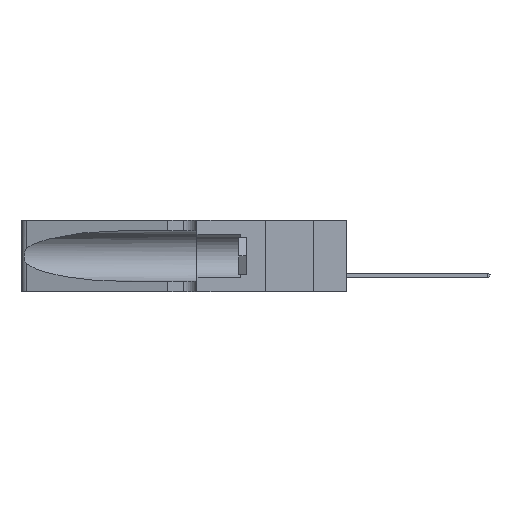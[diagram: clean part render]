
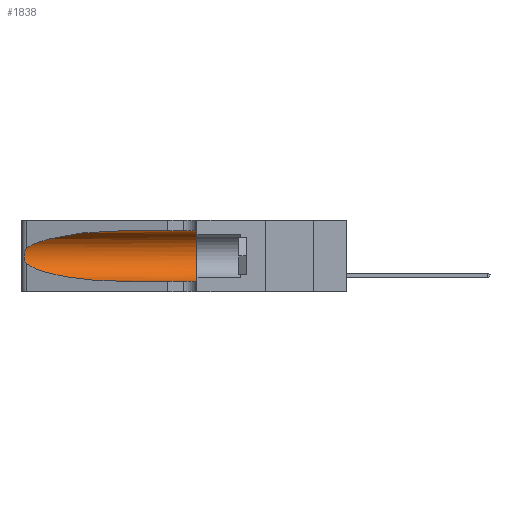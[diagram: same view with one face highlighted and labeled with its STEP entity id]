
A CAD part, left-side view. The second image highlights one B-rep face of the part: STEP entity #1838.
In plain terms, the highlighted cylindrical face has radius 3.308 mm (diameter 6.617 mm), a partial arc.
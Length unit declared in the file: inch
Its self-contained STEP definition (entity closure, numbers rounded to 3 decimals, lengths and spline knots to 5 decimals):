
#1838 = ADVANCED_FACE ( 'NONE', ( #8019 ), #14263, .F. ) ;
#2135 = ORIENTED_EDGE ( 'NONE', *, *, #30698, .F. ) ;
#2615 = CARTESIAN_POINT ( 'NONE',  ( 0.1305, 0.35, 0.05475 ) ) ;
#2997 = CARTESIAN_POINT ( 'NONE',  ( 0.25856, 1.23593, 0.16098 ) ) ;
#3150 = CARTESIAN_POINT ( 'NONE',  ( 0.25854, 1.2359, 0.20912 ) ) ;
#4646 = EDGE_CURVE ( 'NONE', #18827, #30359, #43256, .T. ) ;
#5749 = CARTESIAN_POINT ( 'NONE',  ( 0.25487, 1.22718, 0.22369 ) ) ;
#6407 = VERTEX_POINT ( 'NONE', #25254 ) ;
#6490 = CARTESIAN_POINT ( 'NONE',  ( 0.26075, 1.23896, 0.178 ) ) ;
#8019 = FACE_OUTER_BOUND ( 'NONE', #14316, .T. ) ;
#8082 = CARTESIAN_POINT ( 'NONE',  ( 0.25487, 1.22718, 0.22369 ) ) ;
#8113 = AXIS2_PLACEMENT_3D ( 'NONE', #31915, #13191, #38777 ) ;
#9425 = AXIS2_PLACEMENT_3D ( 'NONE', #25119, #47332, #36017 ) ;
#9522 = VERTEX_POINT ( 'NONE', #5749 ) ;
#11217 = VERTEX_POINT ( 'NONE', #24710 ) ;
#13018 = CARTESIAN_POINT ( 'NONE',  ( 0.25555, 1.22994, 0.2215 ) ) ;
#13031 = CARTESIAN_POINT ( 'NONE',  ( 0.25487, 1.22718, 0.14631 ) ) ;
#13191 = DIRECTION ( 'NONE',  ( 0., 1., 0. ) ) ;
#13321 = CARTESIAN_POINT ( 'NONE',  ( 0.25639, 1.23184, 0.21858 ) ) ;
#13982 = EDGE_CURVE ( 'NONE', #30359, #43902, #23854, .T. ) ;
#14232 =( BOUNDED_CURVE ( )  B_SPLINE_CURVE ( 3, ( #33499, #15241, #44472, #8082 ),
 .UNSPECIFIED., .F., .F. ) 
 B_SPLINE_CURVE_WITH_KNOTS ( ( 4, 4 ),
 ( 1.5708, 2.84003 ),
 .UNSPECIFIED. ) 
 CURVE ( )  GEOMETRIC_REPRESENTATION_ITEM ( )  RATIONAL_B_SPLINE_CURVE ( ( 1., 0.87, 0.87, 1. ) ) 
 REPRESENTATION_ITEM ( '' )  );
#14263 = CYLINDRICAL_SURFACE ( 'NONE', #9425, 0.13025 ) ;
#14316 = EDGE_LOOP ( 'NONE', ( #47153, #45351, #39743, #26605, #2135, #43108 ) ) ;
#15241 = CARTESIAN_POINT ( 'NONE',  ( 0.18966, 0.96281, 0.31525 ) ) ;
#16699 = CARTESIAN_POINT ( 'NONE',  ( 0.18966, 0.96281, 0.05475 ) ) ;
#17005 = CARTESIAN_POINT ( 'NONE',  ( 0.25789, 1.23486, 0.15765 ) ) ;
#17458 = CARTESIAN_POINT ( 'NONE',  ( 0.25487, 1.22718, 0.14631 ) ) ;
#17512 = DIRECTION ( 'NONE',  ( 0., -1., 0. ) ) ;
#18252 = EDGE_CURVE ( 'NONE', #11217, #9522, #14232, .T. ) ;
#18827 = VERTEX_POINT ( 'NONE', #34631 ) ;
#19654 = CIRCLE ( 'NONE', #8113, 0.13025 ) ;
#19898 = CARTESIAN_POINT ( 'NONE',  ( 0.25487, 1.22718, 0.22369 ) ) ;
#20819 = CARTESIAN_POINT ( 'NONE',  ( 0.25555, 1.22993, 0.14849 ) ) ;
#23854 = LINE ( 'NONE', #30295, #34180 ) ;
#24710 = CARTESIAN_POINT ( 'NONE',  ( 0.1305, 0.72297, 0.31525 ) ) ;
#25119 = CARTESIAN_POINT ( 'NONE',  ( 0.1305, 1.61858, 0.185 ) ) ;
#25254 = CARTESIAN_POINT ( 'NONE',  ( 0.1305, 0.35, 0.31525 ) ) ;
#26605 = ORIENTED_EDGE ( 'NONE', *, *, #13982, .T. ) ;
#28659 = CARTESIAN_POINT ( 'NONE',  ( 0.25639, 1.23186, 0.15144 ) ) ;
#28891 = CARTESIAN_POINT ( 'NONE',  ( 0.1305, 1.61858, 0.31525 ) ) ;
#30295 = CARTESIAN_POINT ( 'NONE',  ( 0.1305, 1.61858, 0.05475 ) ) ;
#30359 = VERTEX_POINT ( 'NONE', #31961 ) ;
#30539 = VECTOR ( 'NONE', #17512, 39.37008 ) ;
#30698 = EDGE_CURVE ( 'NONE', #6407, #43902, #19654, .T. ) ;
#31915 = CARTESIAN_POINT ( 'NONE',  ( 0.1305, 0.35, 0.185 ) ) ;
#31961 = CARTESIAN_POINT ( 'NONE',  ( 0.1305, 0.72297, 0.05475 ) ) ;
#32223 = LINE ( 'NONE', #28891, #30539 ) ;
#33499 = CARTESIAN_POINT ( 'NONE',  ( 0.1305, 0.72297, 0.31525 ) ) ;
#34180 = VECTOR ( 'NONE', #37592, 39.37008 ) ;
#34631 = CARTESIAN_POINT ( 'NONE',  ( 0.25487, 1.22718, 0.14631 ) ) ;
#36017 = DIRECTION ( 'NONE',  ( 0., 0., -1. ) ) ;
#36298 = B_SPLINE_CURVE_WITH_KNOTS ( 'NONE', 3,
 ( #19898, #13018, #13321, #43048, #3150, #46243, #38907, #6490, #43184, #2997, #17005, #28659, #20819, #17458 ),
 .UNSPECIFIED., .F., .F.,
 ( 4, 2, 2, 2, 2, 2, 4 ),
 ( 0., 0.00027, 0.00053, 0.00107, 0.0016, 0.00187, 0.00214 ),
 .UNSPECIFIED. ) ;
#37592 = DIRECTION ( 'NONE',  ( 0., -1., 0. ) ) ;
#38564 = EDGE_CURVE ( 'NONE', #11217, #6407, #32223, .T. ) ;
#38777 = DIRECTION ( 'NONE',  ( 0., 0., 1. ) ) ;
#38907 = CARTESIAN_POINT ( 'NONE',  ( 0.26075, 1.23896, 0.19203 ) ) ;
#39012 = EDGE_CURVE ( 'NONE', #9522, #18827, #36298, .T. ) ;
#39743 = ORIENTED_EDGE ( 'NONE', *, *, #4646, .T. ) ;
#42288 = CARTESIAN_POINT ( 'NONE',  ( 0.1305, 0.72297, 0.05475 ) ) ;
#43048 = CARTESIAN_POINT ( 'NONE',  ( 0.25787, 1.23484, 0.2124 ) ) ;
#43108 = ORIENTED_EDGE ( 'NONE', *, *, #38564, .F. ) ;
#43184 = CARTESIAN_POINT ( 'NONE',  ( 0.26017, 1.23833, 0.17102 ) ) ;
#43256 =( BOUNDED_CURVE ( )  B_SPLINE_CURVE ( 3, ( #13031, #46419, #16699, #42288 ),
 .UNSPECIFIED., .F., .T. ) 
 B_SPLINE_CURVE_WITH_KNOTS ( ( 4, 4 ),
 ( 3.44316, 4.71239 ),
 .UNSPECIFIED. ) 
 CURVE ( )  GEOMETRIC_REPRESENTATION_ITEM ( )  RATIONAL_B_SPLINE_CURVE ( ( 1., 0.87, 0.87, 1. ) ) 
 REPRESENTATION_ITEM ( '' )  );
#43902 = VERTEX_POINT ( 'NONE', #2615 ) ;
#44472 = CARTESIAN_POINT ( 'NONE',  ( 0.2373, 1.15595, 0.28018 ) ) ;
#45351 = ORIENTED_EDGE ( 'NONE', *, *, #39012, .T. ) ;
#46243 = CARTESIAN_POINT ( 'NONE',  ( 0.26018, 1.23835, 0.19895 ) ) ;
#46419 = CARTESIAN_POINT ( 'NONE',  ( 0.2373, 1.15595, 0.08982 ) ) ;
#47153 = ORIENTED_EDGE ( 'NONE', *, *, #18252, .T. ) ;
#47332 = DIRECTION ( 'NONE',  ( 0., -1., 0. ) ) ;
